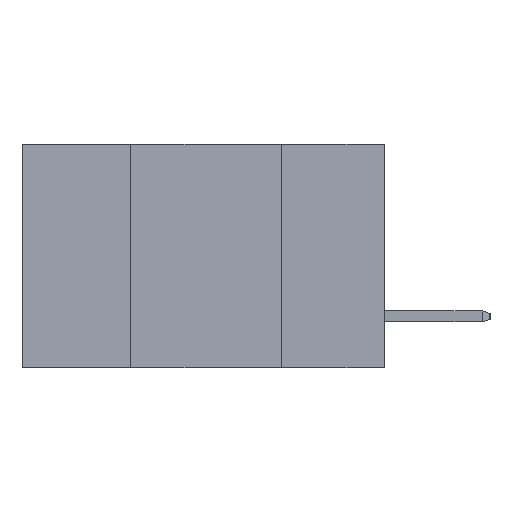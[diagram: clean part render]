
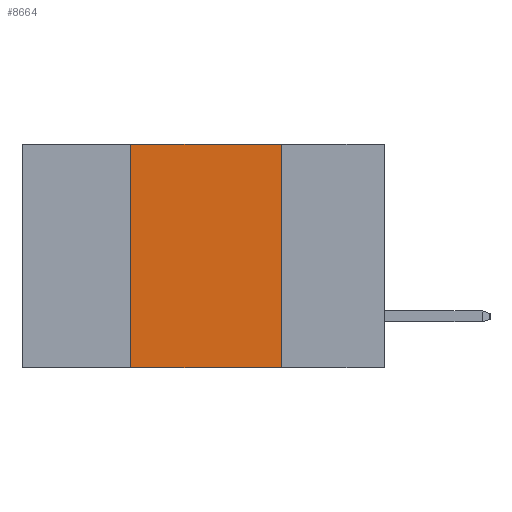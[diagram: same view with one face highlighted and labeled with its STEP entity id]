
A CAD part, left-side view. The second image highlights one B-rep face of the part: STEP entity #8664.
In plain terms, the highlighted planar face has unit normal (-1, 0, 0).
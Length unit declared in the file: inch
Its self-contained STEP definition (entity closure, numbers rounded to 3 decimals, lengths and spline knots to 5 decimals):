
#314 = CARTESIAN_POINT ( 'NONE',  ( 0., 0.6, -0.37 ) ) ;
#521 = EDGE_CURVE ( 'NONE', #24765, #7356, #5675, .T. ) ;
#793 = DIRECTION ( 'NONE',  ( 0., 0., -1. ) ) ;
#2070 = ORIENTED_EDGE ( 'NONE', *, *, #17307, .F. ) ;
#3551 = EDGE_CURVE ( 'NONE', #21007, #21994, #23882, .T. ) ;
#3983 = LINE ( 'NONE', #20770, #20226 ) ;
#4249 = ORIENTED_EDGE ( 'NONE', *, *, #521, .T. ) ;
#5058 = EDGE_LOOP ( 'NONE', ( #2070, #6422, #13503, #4249 ) ) ;
#5675 = LINE ( 'NONE', #314, #20621 ) ;
#5839 = LINE ( 'NONE', #14572, #16276 ) ;
#6422 = ORIENTED_EDGE ( 'NONE', *, *, #3551, .F. ) ;
#7145 = DIRECTION ( 'NONE',  ( 0., 0., 1. ) ) ;
#7356 = VERTEX_POINT ( 'NONE', #10848 ) ;
#8664 = ADVANCED_FACE ( 'NONE', ( #14676 ), #22903, .F. ) ;
#8981 = CARTESIAN_POINT ( 'NONE',  ( 0., 0.6, 0. ) ) ;
#9899 = DIRECTION ( 'NONE',  ( 0., -1., 0. ) ) ;
#10848 = CARTESIAN_POINT ( 'NONE',  ( 0., 0.17, -0.37 ) ) ;
#11359 = DIRECTION ( 'NONE',  ( 1., 0., 0. ) ) ;
#12076 = EDGE_CURVE ( 'NONE', #24765, #21007, #3983, .T. ) ;
#13217 = CARTESIAN_POINT ( 'NONE',  ( 0., 0.6, 0. ) ) ;
#13503 = ORIENTED_EDGE ( 'NONE', *, *, #12076, .F. ) ;
#14572 = CARTESIAN_POINT ( 'NONE',  ( 0., 0.17, 0. ) ) ;
#14676 = FACE_OUTER_BOUND ( 'NONE', #5058, .T. ) ;
#16276 = VECTOR ( 'NONE', #793, 39.37008 ) ;
#17307 = EDGE_CURVE ( 'NONE', #21994, #7356, #5839, .T. ) ;
#18815 = CARTESIAN_POINT ( 'NONE',  ( 0., 0.42, -0.37 ) ) ;
#20226 = VECTOR ( 'NONE', #7145, 39.37008 ) ;
#20621 = VECTOR ( 'NONE', #22039, 39.37008 ) ;
#20770 = CARTESIAN_POINT ( 'NONE',  ( 0., 0.42, 0. ) ) ;
#21007 = VERTEX_POINT ( 'NONE', #24618 ) ;
#21994 = VERTEX_POINT ( 'NONE', #22062 ) ;
#22039 = DIRECTION ( 'NONE',  ( 0., -1., 0. ) ) ;
#22062 = CARTESIAN_POINT ( 'NONE',  ( 0., 0.17, 0. ) ) ;
#22667 = AXIS2_PLACEMENT_3D ( 'NONE', #13217, #11359, #24834 ) ;
#22903 = PLANE ( 'NONE',  #22667 ) ;
#23286 = VECTOR ( 'NONE', #9899, 39.37008 ) ;
#23882 = LINE ( 'NONE', #8981, #23286 ) ;
#24618 = CARTESIAN_POINT ( 'NONE',  ( 0., 0.42, 0. ) ) ;
#24765 = VERTEX_POINT ( 'NONE', #18815 ) ;
#24834 = DIRECTION ( 'NONE',  ( 0., 0., -1. ) ) ;
